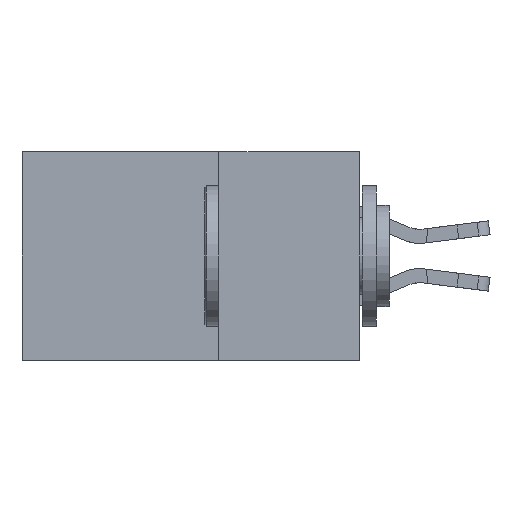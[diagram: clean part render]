
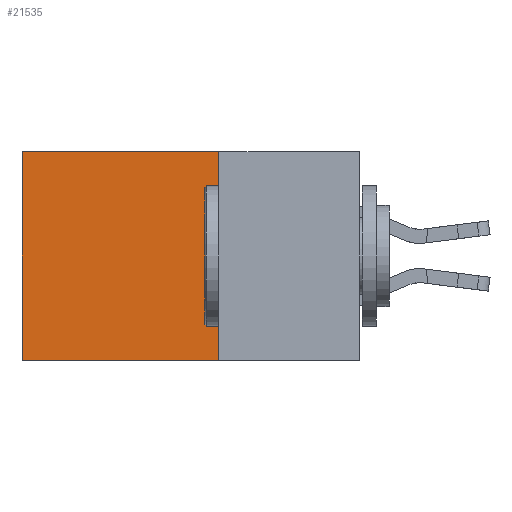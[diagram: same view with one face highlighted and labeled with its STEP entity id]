
A CAD part, left-side view. The second image highlights one B-rep face of the part: STEP entity #21535.
In plain terms, the highlighted planar face has unit normal (-1, 0, 0).
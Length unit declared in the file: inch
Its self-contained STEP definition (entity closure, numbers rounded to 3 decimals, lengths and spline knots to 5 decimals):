
#35 = LINE ( 'NONE', #5532, #2414 ) ;
#449 = VECTOR ( 'NONE', #21103, 39.37008 ) ;
#1070 = VECTOR ( 'NONE', #22620, 39.37008 ) ;
#2333 = EDGE_CURVE ( 'NONE', #5840, #9859, #3056, .T. ) ;
#2414 = VECTOR ( 'NONE', #23979, 39.37008 ) ;
#2498 = FACE_OUTER_BOUND ( 'NONE', #16726, .T. ) ;
#3056 = LINE ( 'NONE', #10946, #11837 ) ;
#4483 = CARTESIAN_POINT ( 'NONE',  ( 0.2875, 0.25, 0. ) ) ;
#5532 = CARTESIAN_POINT ( 'NONE',  ( 0.2875, 0.25, -0.37 ) ) ;
#5717 = CARTESIAN_POINT ( 'NONE',  ( 0.2875, 0.25, 0. ) ) ;
#5840 = VERTEX_POINT ( 'NONE', #9656 ) ;
#6205 = EDGE_CURVE ( 'NONE', #5840, #15966, #12208, .T. ) ;
#9656 = CARTESIAN_POINT ( 'NONE',  ( 0.2875, 0.25, 0. ) ) ;
#9859 = VERTEX_POINT ( 'NONE', #11060 ) ;
#10790 = ORIENTED_EDGE ( 'NONE', *, *, #6205, .F. ) ;
#10946 = CARTESIAN_POINT ( 'NONE',  ( 0.2875, 0.25, 0. ) ) ;
#11060 = CARTESIAN_POINT ( 'NONE',  ( 0.2875, 0.6, 0. ) ) ;
#11837 = VECTOR ( 'NONE', #20239, 39.37008 ) ;
#11907 = EDGE_CURVE ( 'NONE', #9859, #21479, #23549, .T. ) ;
#12208 = LINE ( 'NONE', #5717, #1070 ) ;
#12848 = ORIENTED_EDGE ( 'NONE', *, *, #23713, .F. ) ;
#13910 = PLANE ( 'NONE',  #16629 ) ;
#14323 = CARTESIAN_POINT ( 'NONE',  ( 0.2875, 0.6, -0.37 ) ) ;
#15103 = CARTESIAN_POINT ( 'NONE',  ( 0.2875, 0.6, 0. ) ) ;
#15966 = VERTEX_POINT ( 'NONE', #20989 ) ;
#16016 = DIRECTION ( 'NONE',  ( 1., 0., 0. ) ) ;
#16629 = AXIS2_PLACEMENT_3D ( 'NONE', #4483, #16016, #21375 ) ;
#16711 = ORIENTED_EDGE ( 'NONE', *, *, #2333, .T. ) ;
#16726 = EDGE_LOOP ( 'NONE', ( #17819, #12848, #10790, #16711 ) ) ;
#17819 = ORIENTED_EDGE ( 'NONE', *, *, #11907, .T. ) ;
#20239 = DIRECTION ( 'NONE',  ( 0., 1., 0. ) ) ;
#20989 = CARTESIAN_POINT ( 'NONE',  ( 0.2875, 0.25, -0.37 ) ) ;
#21103 = DIRECTION ( 'NONE',  ( 0., 0., -1. ) ) ;
#21375 = DIRECTION ( 'NONE',  ( 0., 0., -1. ) ) ;
#21479 = VERTEX_POINT ( 'NONE', #14323 ) ;
#21535 = ADVANCED_FACE ( 'NONE', ( #2498 ), #13910, .F. ) ;
#22620 = DIRECTION ( 'NONE',  ( 0., 0., -1. ) ) ;
#23549 = LINE ( 'NONE', #15103, #449 ) ;
#23713 = EDGE_CURVE ( 'NONE', #15966, #21479, #35, .T. ) ;
#23979 = DIRECTION ( 'NONE',  ( 0., 1., 0. ) ) ;
